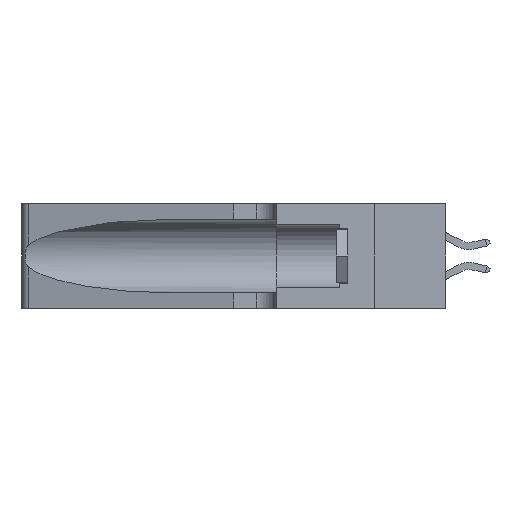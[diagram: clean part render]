
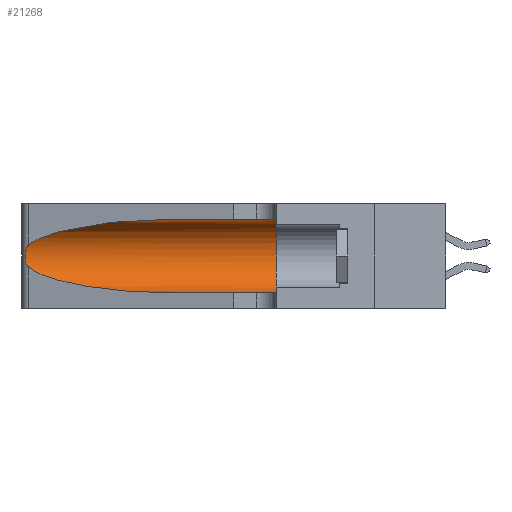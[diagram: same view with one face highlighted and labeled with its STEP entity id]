
A CAD part, left-side view. The second image highlights one B-rep face of the part: STEP entity #21268.
In plain terms, the highlighted cylindrical face has radius 3.308 mm (diameter 6.617 mm), a partial arc.
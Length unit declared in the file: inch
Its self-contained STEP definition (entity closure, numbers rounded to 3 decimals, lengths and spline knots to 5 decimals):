
#393 = EDGE_CURVE ( 'NONE', #25228, #23591, #15332, .T. ) ;
#480 = EDGE_CURVE ( 'NONE', #12595, #25228, #22891, .T. ) ;
#727 = EDGE_LOOP ( 'NONE', ( #3502, #26349, #28343, #23548, #21598, #4673 ) ) ;
#844 = CARTESIAN_POINT ( 'NONE',  ( 0.25854, 1.2359, 0.20912 ) ) ;
#1604 = AXIS2_PLACEMENT_3D ( 'NONE', #26853, #13451, #29107 ) ;
#1641 = EDGE_CURVE ( 'NONE', #8144, #28683, #28072, .T. ) ;
#3202 = CARTESIAN_POINT ( 'NONE',  ( 0.26075, 1.23896, 0.19203 ) ) ;
#3502 = ORIENTED_EDGE ( 'NONE', *, *, #1641, .T. ) ;
#4385 = CARTESIAN_POINT ( 'NONE',  ( 0.1305, 1.61858, 0.185 ) ) ;
#4673 = ORIENTED_EDGE ( 'NONE', *, *, #23073, .F. ) ;
#5489 = CARTESIAN_POINT ( 'NONE',  ( 0.26017, 1.23833, 0.17102 ) ) ;
#5799 = CARTESIAN_POINT ( 'NONE',  ( 0.2373, 1.15595, 0.28018 ) ) ;
#5841 = CARTESIAN_POINT ( 'NONE',  ( 0.1305, 0.72297, 0.31525 ) ) ;
#5867 = B_SPLINE_CURVE_WITH_KNOTS ( 'NONE', 3,
 ( #23544, #14659, #28144, #14759, #844, #17012, #3202, #19262, #5489, #21505, #7818, #23735, #10195, #25997 ),
 .UNSPECIFIED., .F., .F.,
 ( 4, 2, 2, 2, 2, 2, 4 ),
 ( 0., 0.00027, 0.00053, 0.00107, 0.0016, 0.00187, 0.00214 ),
 .UNSPECIFIED. ) ;
#6191 = FACE_OUTER_BOUND ( 'NONE', #727, .T. ) ;
#6441 = CARTESIAN_POINT ( 'NONE',  ( 0.1305, 0.72297, 0.05475 ) ) ;
#6579 = CARTESIAN_POINT ( 'NONE',  ( 0.25487, 1.22718, 0.14631 ) ) ;
#7818 = CARTESIAN_POINT ( 'NONE',  ( 0.25789, 1.23486, 0.15765 ) ) ;
#8144 = VERTEX_POINT ( 'NONE', #22680 ) ;
#10195 = CARTESIAN_POINT ( 'NONE',  ( 0.25555, 1.22993, 0.14849 ) ) ;
#10649 = CARTESIAN_POINT ( 'NONE',  ( 0.1305, 0.72297, 0.05475 ) ) ;
#10861 = CARTESIAN_POINT ( 'NONE',  ( 0.2373, 1.15595, 0.08982 ) ) ;
#12376 = VERTEX_POINT ( 'NONE', #20172 ) ;
#12384 = CARTESIAN_POINT ( 'NONE',  ( 0.18966, 0.96281, 0.05475 ) ) ;
#12595 = VERTEX_POINT ( 'NONE', #14266 ) ;
#12604 = CARTESIAN_POINT ( 'NONE',  ( 0.18966, 0.96281, 0.31525 ) ) ;
#12945 = DIRECTION ( 'NONE',  ( 0., -1., 0. ) ) ;
#12999 = CARTESIAN_POINT ( 'NONE',  ( 0.1305, 1.61858, 0.05475 ) ) ;
#13451 = DIRECTION ( 'NONE',  ( 0., 1., 0. ) ) ;
#13561 = EDGE_CURVE ( 'NONE', #12376, #23591, #22085, .T. ) ;
#13664 = DIRECTION ( 'NONE',  ( 0., -1., 0. ) ) ;
#13842 = CARTESIAN_POINT ( 'NONE',  ( 0.25487, 1.22718, 0.22369 ) ) ;
#14266 = CARTESIAN_POINT ( 'NONE',  ( 0.25487, 1.22718, 0.14631 ) ) ;
#14658 = VECTOR ( 'NONE', #19631, 39.37008 ) ;
#14659 = CARTESIAN_POINT ( 'NONE',  ( 0.25555, 1.22994, 0.2215 ) ) ;
#14759 = CARTESIAN_POINT ( 'NONE',  ( 0.25787, 1.23484, 0.2124 ) ) ;
#15332 = LINE ( 'NONE', #12999, #27938 ) ;
#15880 = CARTESIAN_POINT ( 'NONE',  ( 0.1305, 0.35, 0.05475 ) ) ;
#16093 = AXIS2_PLACEMENT_3D ( 'NONE', #4385, #13664, #20425 ) ;
#17012 = CARTESIAN_POINT ( 'NONE',  ( 0.26018, 1.23835, 0.19895 ) ) ;
#17917 = EDGE_CURVE ( 'NONE', #28683, #12595, #5867, .T. ) ;
#19033 = CARTESIAN_POINT ( 'NONE',  ( 0.25487, 1.22718, 0.22369 ) ) ;
#19262 = CARTESIAN_POINT ( 'NONE',  ( 0.26075, 1.23896, 0.178 ) ) ;
#19631 = DIRECTION ( 'NONE',  ( 0., -1., 0. ) ) ;
#20172 = CARTESIAN_POINT ( 'NONE',  ( 0.1305, 0.35, 0.31525 ) ) ;
#20425 = DIRECTION ( 'NONE',  ( 0., 0., -1. ) ) ;
#20622 = LINE ( 'NONE', #28535, #14658 ) ;
#21268 = ADVANCED_FACE ( 'NONE', ( #6191 ), #23679, .F. ) ;
#21505 = CARTESIAN_POINT ( 'NONE',  ( 0.25856, 1.23593, 0.16098 ) ) ;
#21598 = ORIENTED_EDGE ( 'NONE', *, *, #13561, .F. ) ;
#22085 = CIRCLE ( 'NONE', #1604, 0.13025 ) ;
#22680 = CARTESIAN_POINT ( 'NONE',  ( 0.1305, 0.72297, 0.31525 ) ) ;
#22891 =( BOUNDED_CURVE ( )  B_SPLINE_CURVE ( 3, ( #6579, #10861, #12384, #6441 ),
 .UNSPECIFIED., .F., .F. ) 
 B_SPLINE_CURVE_WITH_KNOTS ( ( 4, 4 ),
 ( 3.44316, 4.71239 ),
 .UNSPECIFIED. ) 
 CURVE ( )  GEOMETRIC_REPRESENTATION_ITEM ( )  RATIONAL_B_SPLINE_CURVE ( ( 1., 0.87, 0.87, 1. ) ) 
 REPRESENTATION_ITEM ( '' )  );
#23073 = EDGE_CURVE ( 'NONE', #8144, #12376, #20622, .T. ) ;
#23544 = CARTESIAN_POINT ( 'NONE',  ( 0.25487, 1.22718, 0.22369 ) ) ;
#23548 = ORIENTED_EDGE ( 'NONE', *, *, #393, .T. ) ;
#23591 = VERTEX_POINT ( 'NONE', #15880 ) ;
#23679 = CYLINDRICAL_SURFACE ( 'NONE', #16093, 0.13025 ) ;
#23735 = CARTESIAN_POINT ( 'NONE',  ( 0.25639, 1.23186, 0.15144 ) ) ;
#25228 = VERTEX_POINT ( 'NONE', #10649 ) ;
#25997 = CARTESIAN_POINT ( 'NONE',  ( 0.25487, 1.22718, 0.14631 ) ) ;
#26349 = ORIENTED_EDGE ( 'NONE', *, *, #17917, .T. ) ;
#26853 = CARTESIAN_POINT ( 'NONE',  ( 0.1305, 0.35, 0.185 ) ) ;
#27938 = VECTOR ( 'NONE', #12945, 39.37008 ) ;
#28072 =( BOUNDED_CURVE ( )  B_SPLINE_CURVE ( 3, ( #5841, #12604, #5799, #19033 ),
 .UNSPECIFIED., .F., .T. ) 
 B_SPLINE_CURVE_WITH_KNOTS ( ( 4, 4 ),
 ( 1.5708, 2.84003 ),
 .UNSPECIFIED. ) 
 CURVE ( )  GEOMETRIC_REPRESENTATION_ITEM ( )  RATIONAL_B_SPLINE_CURVE ( ( 1., 0.87, 0.87, 1. ) ) 
 REPRESENTATION_ITEM ( '' )  );
#28144 = CARTESIAN_POINT ( 'NONE',  ( 0.25639, 1.23184, 0.21858 ) ) ;
#28343 = ORIENTED_EDGE ( 'NONE', *, *, #480, .T. ) ;
#28535 = CARTESIAN_POINT ( 'NONE',  ( 0.1305, 1.61858, 0.31525 ) ) ;
#28683 = VERTEX_POINT ( 'NONE', #13842 ) ;
#29107 = DIRECTION ( 'NONE',  ( 0., 0., 1. ) ) ;
